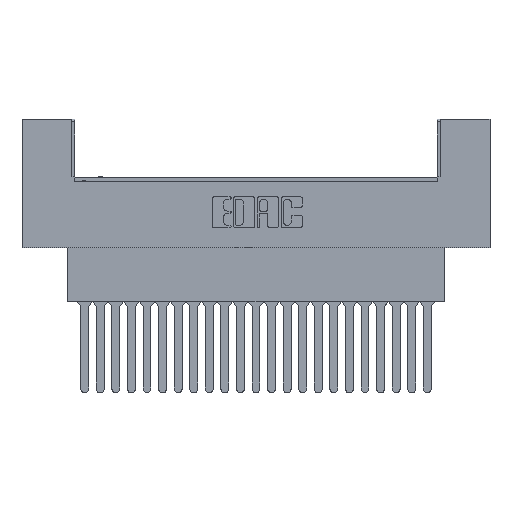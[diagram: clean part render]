
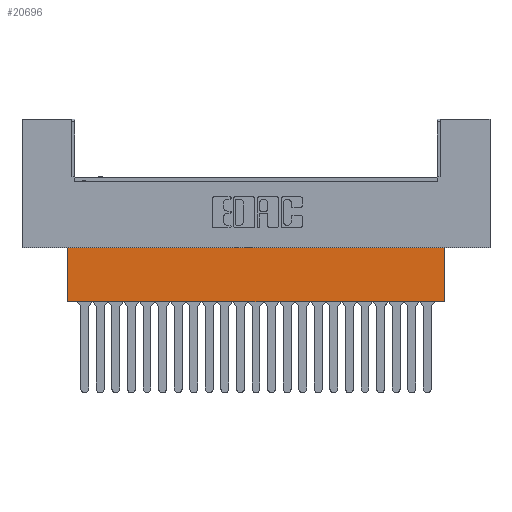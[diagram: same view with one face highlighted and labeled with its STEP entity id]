
A CAD part, top view. The second image highlights one B-rep face of the part: STEP entity #20696.
In plain terms, the highlighted planar face has unit normal (0, 0, 1).
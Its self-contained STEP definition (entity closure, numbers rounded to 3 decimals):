
#1098 = VERTEX_POINT ( 'NONE', #28565 ) ;
#1122 = CARTESIAN_POINT ( 'NONE',  ( 68.885, 0., -3.962 ) ) ;
#1200 = PLANE ( 'NONE',  #26369 ) ;
#1544 = EDGE_CURVE ( 'NONE', #11643, #1098, #8034, .T. ) ;
#3016 = VECTOR ( 'NONE', #10155, 1000. ) ;
#4710 = CARTESIAN_POINT ( 'NONE',  ( 68.885, -8.814, -3.962 ) ) ;
#4828 = EDGE_LOOP ( 'NONE', ( #28703, #14352, #8267, #10778 ) ) ;
#5470 = EDGE_CURVE ( 'NONE', #11643, #19624, #13838, .T. ) ;
#6376 = DIRECTION ( 'NONE',  ( 0., 1., 0. ) ) ;
#7201 = VECTOR ( 'NONE', #17552, 1000. ) ;
#7874 = CARTESIAN_POINT ( 'NONE',  ( 76.352, 0., -3.962 ) ) ;
#8034 = LINE ( 'NONE', #26637, #14886 ) ;
#8267 = ORIENTED_EDGE ( 'NONE', *, *, #1544, .T. ) ;
#8385 = CARTESIAN_POINT ( 'NONE',  ( 76.352, -8.814, -3.962 ) ) ;
#10155 = DIRECTION ( 'NONE',  ( 0., -1., 0. ) ) ;
#10259 = CARTESIAN_POINT ( 'NONE',  ( 68.885, -8.814, -3.962 ) ) ;
#10778 = ORIENTED_EDGE ( 'NONE', *, *, #12526, .F. ) ;
#11643 = VERTEX_POINT ( 'NONE', #1122 ) ;
#12526 = EDGE_CURVE ( 'NONE', #15219, #1098, #27703, .T. ) ;
#13838 = LINE ( 'NONE', #10259, #3016 ) ;
#14352 = ORIENTED_EDGE ( 'NONE', *, *, #5470, .F. ) ;
#14829 = DIRECTION ( 'NONE',  ( 0., 0., -1. ) ) ;
#14886 = VECTOR ( 'NONE', #28726, 1000. ) ;
#15219 = VERTEX_POINT ( 'NONE', #22977 ) ;
#17537 = EDGE_CURVE ( 'NONE', #19624, #15219, #25193, .T. ) ;
#17552 = DIRECTION ( 'NONE',  ( -1., 0., 0. ) ) ;
#19624 = VERTEX_POINT ( 'NONE', #4710 ) ;
#20696 = ADVANCED_FACE ( 'NONE', ( #25788 ), #1200, .F. ) ;
#21870 = DIRECTION ( 'NONE',  ( 0., 1., 0. ) ) ;
#22977 = CARTESIAN_POINT ( 'NONE',  ( 7.468, -8.814, -3.962 ) ) ;
#24688 = CARTESIAN_POINT ( 'NONE',  ( 7.468, -8.814, -3.962 ) ) ;
#25193 = LINE ( 'NONE', #8385, #7201 ) ;
#25788 = FACE_OUTER_BOUND ( 'NONE', #4828, .T. ) ;
#26369 = AXIS2_PLACEMENT_3D ( 'NONE', #7874, #14829, #21870 ) ;
#26637 = CARTESIAN_POINT ( 'NONE',  ( 76.352, 0., -3.962 ) ) ;
#26986 = VECTOR ( 'NONE', #6376, 1000. ) ;
#27703 = LINE ( 'NONE', #24688, #26986 ) ;
#28565 = CARTESIAN_POINT ( 'NONE',  ( 7.468, 0., -3.962 ) ) ;
#28703 = ORIENTED_EDGE ( 'NONE', *, *, #17537, .F. ) ;
#28726 = DIRECTION ( 'NONE',  ( -1., 0., 0. ) ) ;
